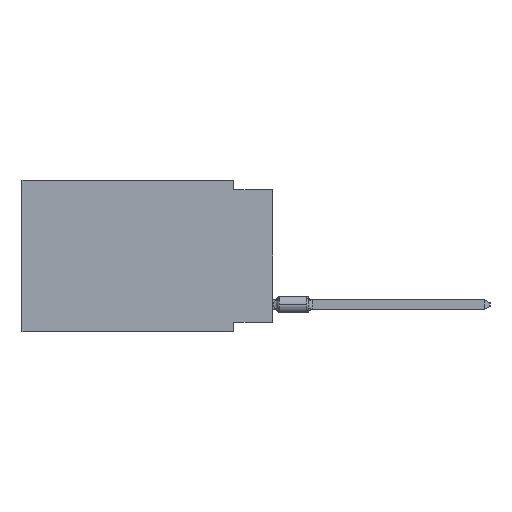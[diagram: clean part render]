
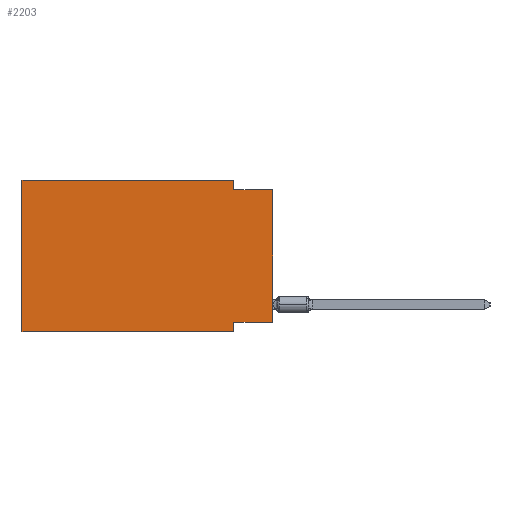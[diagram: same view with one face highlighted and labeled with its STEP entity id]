
A CAD part, left-side view. The second image highlights one B-rep face of the part: STEP entity #2203.
In plain terms, the highlighted planar face has unit normal (-1, 0, 0).
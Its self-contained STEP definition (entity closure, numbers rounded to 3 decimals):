
#647 = CARTESIAN_POINT ( 'NONE',  ( 0., 0., 0. ) ) ;
#1431 = CARTESIAN_POINT ( 'NONE',  ( 0., 16.383, 0. ) ) ;
#1932 = CARTESIAN_POINT ( 'NONE',  ( 0., 16.383, 0. ) ) ;
#2178 = DIRECTION ( 'NONE',  ( 1., 0., 0. ) ) ;
#2203 = ADVANCED_FACE ( 'NONE', ( #25823 ), #22616, .F. ) ;
#2922 = VECTOR ( 'NONE', #9026, 1000. ) ;
#4489 = VECTOR ( 'NONE', #16580, 1000. ) ;
#4553 = VERTEX_POINT ( 'NONE', #14676 ) ;
#5017 = CARTESIAN_POINT ( 'NONE',  ( 0., 0., -0.635 ) ) ;
#5577 = ORIENTED_EDGE ( 'NONE', *, *, #8679, .F. ) ;
#5978 = VERTEX_POINT ( 'NONE', #36575 ) ;
#6211 = DIRECTION ( 'NONE',  ( 0., 1., 0. ) ) ;
#6383 = EDGE_CURVE ( 'NONE', #30904, #5978, #8131, .T. ) ;
#6465 = VERTEX_POINT ( 'NONE', #31604 ) ;
#6539 = LINE ( 'NONE', #20398, #2922 ) ;
#6708 = EDGE_CURVE ( 'NONE', #17226, #27201, #19644, .T. ) ;
#7143 = ORIENTED_EDGE ( 'NONE', *, *, #18385, .T. ) ;
#8131 = LINE ( 'NONE', #16285, #33152 ) ;
#8645 = ORIENTED_EDGE ( 'NONE', *, *, #26271, .T. ) ;
#8679 = EDGE_CURVE ( 'NONE', #17012, #6465, #6539, .T. ) ;
#8884 = LINE ( 'NONE', #12277, #11234 ) ;
#9020 = CARTESIAN_POINT ( 'NONE',  ( 0., 2.54, -9.271 ) ) ;
#9026 = DIRECTION ( 'NONE',  ( 0., 0., -1. ) ) ;
#10267 = DIRECTION ( 'NONE',  ( 0., -1., 0. ) ) ;
#10294 = ORIENTED_EDGE ( 'NONE', *, *, #23705, .F. ) ;
#10703 = DIRECTION ( 'NONE',  ( 0., 0., -1. ) ) ;
#11234 = VECTOR ( 'NONE', #6211, 1000. ) ;
#12277 = CARTESIAN_POINT ( 'NONE',  ( 0., 0., -9.271 ) ) ;
#12609 = VECTOR ( 'NONE', #33656, 1000. ) ;
#12735 = LINE ( 'NONE', #36192, #27022 ) ;
#13089 = ORIENTED_EDGE ( 'NONE', *, *, #21454, .F. ) ;
#13676 = DIRECTION ( 'NONE',  ( 0., -1., 0. ) ) ;
#14676 = CARTESIAN_POINT ( 'NONE',  ( 0., 0., -9.271 ) ) ;
#16285 = CARTESIAN_POINT ( 'NONE',  ( 0., 2.54, 0. ) ) ;
#16580 = DIRECTION ( 'NONE',  ( 0., -1., 0. ) ) ;
#17012 = VERTEX_POINT ( 'NONE', #9020 ) ;
#17145 = VECTOR ( 'NONE', #18081, 1000. ) ;
#17226 = VERTEX_POINT ( 'NONE', #35138 ) ;
#18081 = DIRECTION ( 'NONE',  ( 0., 0., 1. ) ) ;
#18180 = CARTESIAN_POINT ( 'NONE',  ( 0., 2.54, 0. ) ) ;
#18385 = EDGE_CURVE ( 'NONE', #4553, #18813, #26584, .T. ) ;
#18813 = VERTEX_POINT ( 'NONE', #30417 ) ;
#18912 = EDGE_CURVE ( 'NONE', #5978, #18813, #37189, .T. ) ;
#19644 = LINE ( 'NONE', #25121, #12609 ) ;
#20118 = ORIENTED_EDGE ( 'NONE', *, *, #6383, .F. ) ;
#20398 = CARTESIAN_POINT ( 'NONE',  ( 0., 2.54, -9.906 ) ) ;
#21454 = EDGE_CURVE ( 'NONE', #4553, #17012, #8884, .T. ) ;
#21927 = EDGE_LOOP ( 'NONE', ( #7143, #28670, #20118, #10294, #30470, #8645, #5577, #13089 ) ) ;
#22616 = PLANE ( 'NONE',  #32942 ) ;
#23705 = EDGE_CURVE ( 'NONE', #27201, #30904, #31466, .T. ) ;
#24983 = DIRECTION ( 'NONE',  ( 0., 0., -1. ) ) ;
#25082 = CARTESIAN_POINT ( 'NONE',  ( 0., 16.383, 0. ) ) ;
#25121 = CARTESIAN_POINT ( 'NONE',  ( 0., 16.383, 0. ) ) ;
#25823 = FACE_OUTER_BOUND ( 'NONE', #21927, .T. ) ;
#26271 = EDGE_CURVE ( 'NONE', #17226, #6465, #12735, .T. ) ;
#26584 = LINE ( 'NONE', #647, #17145 ) ;
#27022 = VECTOR ( 'NONE', #10267, 1000. ) ;
#27201 = VERTEX_POINT ( 'NONE', #1431 ) ;
#28670 = ORIENTED_EDGE ( 'NONE', *, *, #18912, .F. ) ;
#30417 = CARTESIAN_POINT ( 'NONE',  ( 0., 0., -0.635 ) ) ;
#30470 = ORIENTED_EDGE ( 'NONE', *, *, #6708, .F. ) ;
#30904 = VERTEX_POINT ( 'NONE', #18180 ) ;
#31466 = LINE ( 'NONE', #1932, #32781 ) ;
#31604 = CARTESIAN_POINT ( 'NONE',  ( 0., 2.54, -9.906 ) ) ;
#32781 = VECTOR ( 'NONE', #13676, 1000. ) ;
#32942 = AXIS2_PLACEMENT_3D ( 'NONE', #25082, #2178, #10703 ) ;
#33152 = VECTOR ( 'NONE', #24983, 1000. ) ;
#33656 = DIRECTION ( 'NONE',  ( 0., 0., 1. ) ) ;
#35138 = CARTESIAN_POINT ( 'NONE',  ( 0., 16.383, -9.906 ) ) ;
#36192 = CARTESIAN_POINT ( 'NONE',  ( 0., 16.383, -9.906 ) ) ;
#36575 = CARTESIAN_POINT ( 'NONE',  ( 0., 2.54, -0.635 ) ) ;
#37189 = LINE ( 'NONE', #5017, #4489 ) ;
